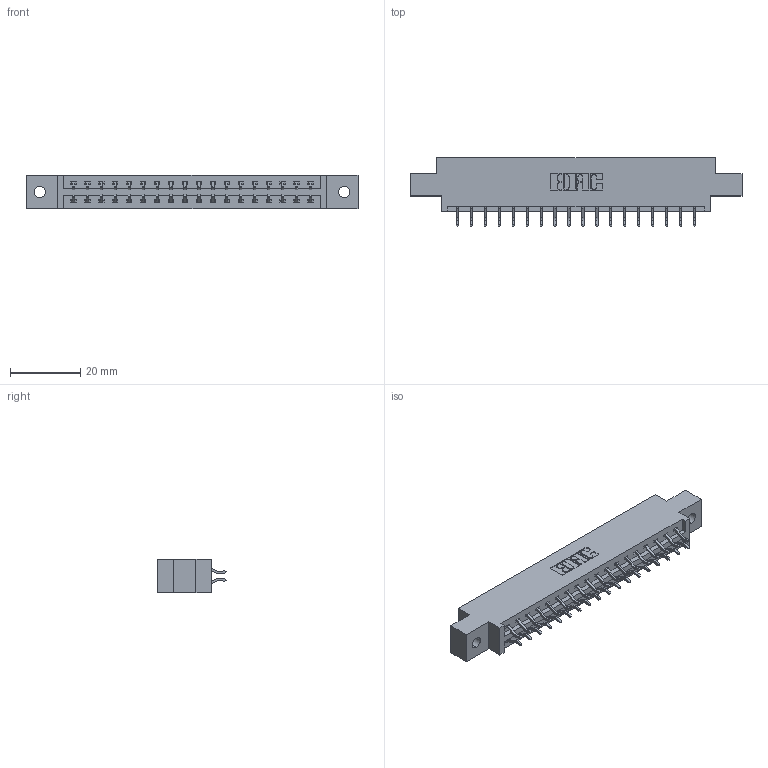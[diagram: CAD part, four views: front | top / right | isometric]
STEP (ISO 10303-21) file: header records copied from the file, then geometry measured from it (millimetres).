
FILE_DESCRIPTION (( 'STEP AP203' ), '1' );
FILE_NAME ('337-036-556-802.STEP', '2018-08-07T23:53:20', ( '' ), ( '' ), 'SwSTEP 2.0', 'SolidWorks 2016', '' );
FILE_SCHEMA (( 'CONFIG_CONTROL_DESIGN' ));
Length unit declared in the file: inch
Products named in the file (3): 337 Part_0.170 Offset - 0.128 Dia; 345-292-001_556 Tail; 337-036-556-802
Assembly tree (37 placements, depth 2):
  337-036-556-802
    337 Part_0.170 Offset - 0.128 Dia
    345-292-001_556 Tail  x36
Bounding box: 94.34 x 19.57 x 9.4 mm (x, y, z)
Volume: 9466.8 mm3; surface area: 10266.2 mm2
Topology: 37 solids, 37 shells, 2278 faces, 6767 edges, 4462 vertices
Faces by surface type: plane 1586, cylinder 692
Entity records: 17415 total; most frequent: CARTESIAN_POINT 2970, ORIENTED_EDGE 2894, DIRECTION 2559, EDGE_CURVE 1447, LINE 1311, VECTOR 1311, VERTEX_POINT 962, AXIS2_PLACEMENT_3D 624
